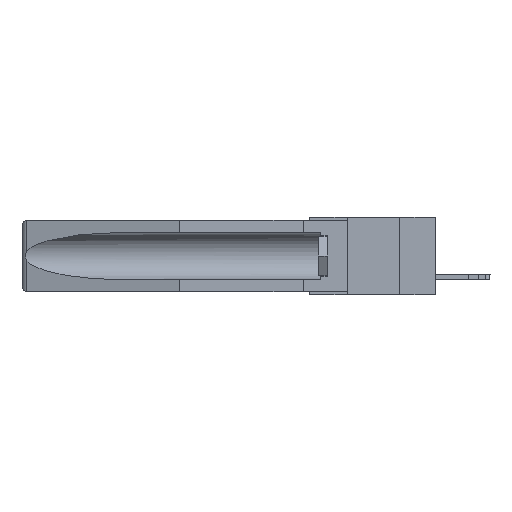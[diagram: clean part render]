
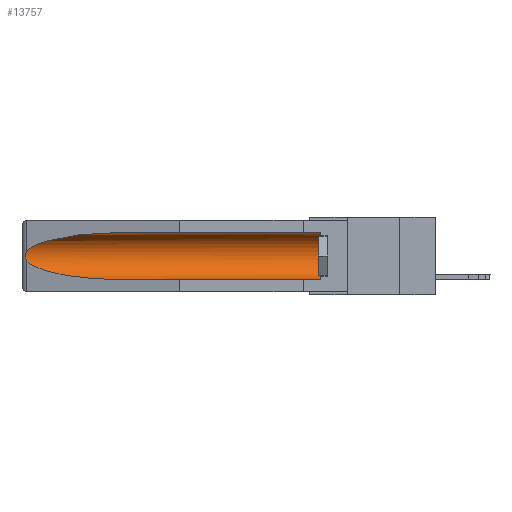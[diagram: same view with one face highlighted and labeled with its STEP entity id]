
A CAD part, left-side view. The second image highlights one B-rep face of the part: STEP entity #13757.
In plain terms, the highlighted cylindrical face has radius 2.857 mm (diameter 5.715 mm), a partial arc.
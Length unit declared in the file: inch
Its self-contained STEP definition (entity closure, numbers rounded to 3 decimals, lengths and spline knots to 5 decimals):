
#976 = CARTESIAN_POINT ( 'NONE',  ( 0.21114, 1.30732, -0.284 ) ) ;
#1296 = FACE_OUTER_BOUND ( 'NONE', #13775, .T. ) ;
#1657 = CARTESIAN_POINT ( 'NONE',  ( 0.155, 0.126, -0.059 ) ) ;
#1752 = CARTESIAN_POINT ( 'NONE',  ( 0.26654, 1.53092, -0.15636 ) ) ;
#1813 = CARTESIAN_POINT ( 'NONE',  ( 0.2673, 1.5327, -0.16383 ) ) ;
#2083 = ORIENTED_EDGE ( 'NONE', *, *, #5034, .T. ) ;
#2333 = CARTESIAN_POINT ( 'NONE',  ( 0.26537, 1.52718, -0.14972 ) ) ;
#2774 = CARTESIAN_POINT ( 'NONE',  ( 0.155, -0.30754, -0.284 ) ) ;
#3246 = EDGE_CURVE ( 'NONE', #5617, #17896, #13258, .T. ) ;
#3504 = CARTESIAN_POINT ( 'NONE',  ( 0.26537, 1.52718, -0.19328 ) ) ;
#3535 = DIRECTION ( 'NONE',  ( 0., 1., 0. ) ) ;
#4135 = CARTESIAN_POINT ( 'NONE',  ( 0.26537, 1.52718, -0.19328 ) ) ;
#4252 = EDGE_CURVE ( 'NONE', #16255, #12525, #4636, .T. ) ;
#4494 = AXIS2_PLACEMENT_3D ( 'NONE', #19112, #3535, #14511 ) ;
#4514 = CARTESIAN_POINT ( 'NONE',  ( 0.155, -0.30754, -0.059 ) ) ;
#4636 = LINE ( 'NONE', #4514, #14423 ) ;
#4974 = CARTESIAN_POINT ( 'NONE',  ( 0.26655, 1.53094, -0.18657 ) ) ;
#5034 = EDGE_CURVE ( 'NONE', #12525, #5617, #17275, .T. ) ;
#5286 = VERTEX_POINT ( 'NONE', #9993 ) ;
#5617 = VERTEX_POINT ( 'NONE', #2333 ) ;
#5653 = CARTESIAN_POINT ( 'NONE',  ( 0.26537, 1.52718, -0.14972 ) ) ;
#6007 = CIRCLE ( 'NONE', #12595, 0.1125 ) ;
#6207 = LINE ( 'NONE', #2774, #10619 ) ;
#6463 = CARTESIAN_POINT ( 'NONE',  ( 0.2675, 1.53308, -0.17534 ) ) ;
#6754 = EDGE_CURVE ( 'NONE', #17896, #8125, #19241, .T. ) ;
#7185 = CARTESIAN_POINT ( 'NONE',  ( 0.155, 1.07973, -0.284 ) ) ;
#7950 = CARTESIAN_POINT ( 'NONE',  ( 0.26597, 1.52961, -0.15275 ) ) ;
#8125 = VERTEX_POINT ( 'NONE', #13946 ) ;
#8485 = ORIENTED_EDGE ( 'NONE', *, *, #6754, .T. ) ;
#8793 = CARTESIAN_POINT ( 'NONE',  ( 0.26537, 1.52718, -0.19328 ) ) ;
#9664 = CARTESIAN_POINT ( 'NONE',  ( 0.26597, 1.5296, -0.19026 ) ) ;
#9944 = ORIENTED_EDGE ( 'NONE', *, *, #4252, .T. ) ;
#9993 = CARTESIAN_POINT ( 'NONE',  ( 0.155, 0.126, -0.284 ) ) ;
#10612 = DIRECTION ( 'NONE',  ( 0., -1., 0. ) ) ;
#10619 = VECTOR ( 'NONE', #13436, 39.37008 ) ;
#11723 = CARTESIAN_POINT ( 'NONE',  ( 0.25451, 1.48313, -0.24835 ) ) ;
#11937 = CARTESIAN_POINT ( 'NONE',  ( 0.21114, 1.30732, -0.059 ) ) ;
#12525 = VERTEX_POINT ( 'NONE', #18682 ) ;
#12580 = EDGE_CURVE ( 'NONE', #5286, #16255, #6007, .T. ) ;
#12595 = AXIS2_PLACEMENT_3D ( 'NONE', #19916, #10612, #15327 ) ;
#12627 = CARTESIAN_POINT ( 'NONE',  ( 0.26537, 1.52718, -0.14972 ) ) ;
#12893 = ORIENTED_EDGE ( 'NONE', *, *, #3246, .T. ) ;
#13258 = B_SPLINE_CURVE_WITH_KNOTS ( 'NONE', 3,
 ( #12627, #7950, #1752, #1813, #15832, #6463, #15895, #4974, #9664, #3504 ),
 .UNSPECIFIED., .F., .F.,
 ( 4, 2, 2, 2, 4 ),
 ( 0., 0.00029, 0.00058, 0.00087, 0.00117 ),
 .UNSPECIFIED. ) ;
#13349 = EDGE_CURVE ( 'NONE', #5286, #8125, #6207, .T. ) ;
#13436 = DIRECTION ( 'NONE',  ( 0., 1., 0. ) ) ;
#13499 = CARTESIAN_POINT ( 'NONE',  ( 0.25451, 1.48313, -0.09465 ) ) ;
#13757 = ADVANCED_FACE ( 'NONE', ( #1296 ), #17205, .F. ) ;
#13775 = EDGE_LOOP ( 'NONE', ( #2083, #12893, #8485, #14339, #17246, #9944 ) ) ;
#13946 = CARTESIAN_POINT ( 'NONE',  ( 0.155, 1.07973, -0.284 ) ) ;
#14339 = ORIENTED_EDGE ( 'NONE', *, *, #13349, .F. ) ;
#14423 = VECTOR ( 'NONE', #18444, 39.37008 ) ;
#14511 = DIRECTION ( 'NONE',  ( 0., 0., 1. ) ) ;
#15078 = CARTESIAN_POINT ( 'NONE',  ( 0.155, 1.07973, -0.059 ) ) ;
#15327 = DIRECTION ( 'NONE',  ( 0., 0., 1. ) ) ;
#15832 = CARTESIAN_POINT ( 'NONE',  ( 0.2675, 1.53308, -0.16763 ) ) ;
#15895 = CARTESIAN_POINT ( 'NONE',  ( 0.2673, 1.53269, -0.17917 ) ) ;
#16255 = VERTEX_POINT ( 'NONE', #1657 ) ;
#17205 = CYLINDRICAL_SURFACE ( 'NONE', #4494, 0.1125 ) ;
#17246 = ORIENTED_EDGE ( 'NONE', *, *, #12580, .T. ) ;
#17275 =( BOUNDED_CURVE ( )  B_SPLINE_CURVE ( 3, ( #15078, #11937, #13499, #5653 ),
 .UNSPECIFIED., .F., .F. ) 
 B_SPLINE_CURVE_WITH_KNOTS ( ( 4, 4 ),
 ( 4.71239, 6.08839 ),
 .UNSPECIFIED. ) 
 CURVE ( )  GEOMETRIC_REPRESENTATION_ITEM ( )  RATIONAL_B_SPLINE_CURVE ( ( 1., 0.848, 0.848, 1. ) ) 
 REPRESENTATION_ITEM ( '' )  );
#17896 = VERTEX_POINT ( 'NONE', #8793 ) ;
#18444 = DIRECTION ( 'NONE',  ( 0., 1., 0. ) ) ;
#18682 = CARTESIAN_POINT ( 'NONE',  ( 0.155, 1.07973, -0.059 ) ) ;
#19112 = CARTESIAN_POINT ( 'NONE',  ( 0.155, -0.30754, -0.1715 ) ) ;
#19241 =( BOUNDED_CURVE ( )  B_SPLINE_CURVE ( 3, ( #4135, #11723, #976, #7185 ),
 .UNSPECIFIED., .F., .F. ) 
 B_SPLINE_CURVE_WITH_KNOTS ( ( 4, 4 ),
 ( 0.1948, 1.5708 ),
 .UNSPECIFIED. ) 
 CURVE ( )  GEOMETRIC_REPRESENTATION_ITEM ( )  RATIONAL_B_SPLINE_CURVE ( ( 1., 0.848, 0.848, 1. ) ) 
 REPRESENTATION_ITEM ( '' )  );
#19916 = CARTESIAN_POINT ( 'NONE',  ( 0.155, 0.126, -0.1715 ) ) ;
